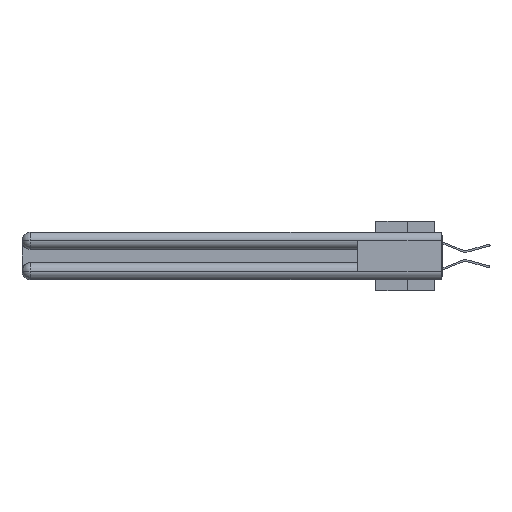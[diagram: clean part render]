
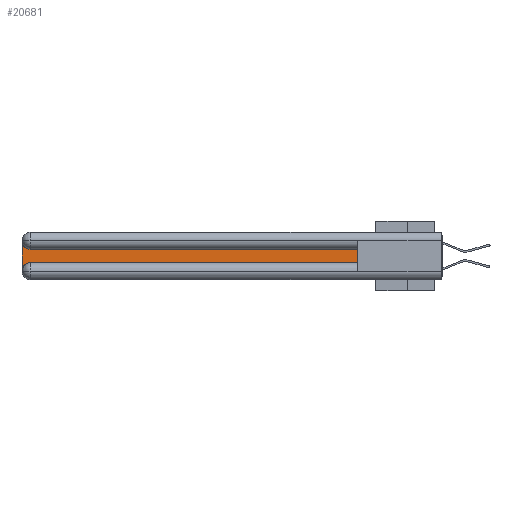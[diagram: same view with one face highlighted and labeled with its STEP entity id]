
A CAD part, left-side view. The second image highlights one B-rep face of the part: STEP entity #20681.
In plain terms, the highlighted planar face has unit normal (-1, 0, 0).
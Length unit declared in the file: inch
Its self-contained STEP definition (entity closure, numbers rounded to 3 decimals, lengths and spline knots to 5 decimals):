
#6 = ORIENTED_EDGE ( 'NONE', *, *, #23174, .T. ) ;
#314 = CIRCLE ( 'NONE', #15308, 0.06 ) ;
#1914 = CARTESIAN_POINT ( 'NONE',  ( 0.075, 2.94, -0.1225 ) ) ;
#2715 = CARTESIAN_POINT ( 'NONE',  ( 0.075, 0.6, -0.2175 ) ) ;
#2827 = DIRECTION ( 'NONE',  ( 1., 0., 0. ) ) ;
#3104 = VERTEX_POINT ( 'NONE', #15729 ) ;
#3452 = CARTESIAN_POINT ( 'NONE',  ( 0.075, 2.94, -0.2775 ) ) ;
#5045 = EDGE_CURVE ( 'NONE', #33990, #6914, #17388, .T. ) ;
#5106 = DIRECTION ( 'NONE',  ( 0., 0., 1. ) ) ;
#5111 = ORIENTED_EDGE ( 'NONE', *, *, #5045, .T. ) ;
#5476 = CARTESIAN_POINT ( 'NONE',  ( 0.075, 0.6, -0.2175 ) ) ;
#5692 = VERTEX_POINT ( 'NONE', #2715 ) ;
#6135 = EDGE_CURVE ( 'NONE', #6914, #3104, #15519, .T. ) ;
#6412 = EDGE_LOOP ( 'NONE', ( #8055, #5111, #7469, #12087, #20218, #6 ) ) ;
#6914 = VERTEX_POINT ( 'NONE', #10956 ) ;
#7347 = DIRECTION ( 'NONE',  ( 0., 1., 0. ) ) ;
#7469 = ORIENTED_EDGE ( 'NONE', *, *, #6135, .T. ) ;
#7632 = EDGE_CURVE ( 'NONE', #3104, #33728, #314, .T. ) ;
#7634 = DIRECTION ( 'NONE',  ( 0., 0., -1. ) ) ;
#8055 = ORIENTED_EDGE ( 'NONE', *, *, #29103, .T. ) ;
#8430 = VERTEX_POINT ( 'NONE', #36486 ) ;
#8545 = VECTOR ( 'NONE', #36013, 39.37008 ) ;
#8676 = FACE_OUTER_BOUND ( 'NONE', #6412, .T. ) ;
#10293 = LINE ( 'NONE', #18914, #13581 ) ;
#10956 = CARTESIAN_POINT ( 'NONE',  ( 0.075, 3., -0.0625 ) ) ;
#11819 = CARTESIAN_POINT ( 'NONE',  ( 0.075, 3., -0.1225 ) ) ;
#12087 = ORIENTED_EDGE ( 'NONE', *, *, #7632, .T. ) ;
#12193 = DIRECTION ( 'NONE',  ( 0., 0., -1. ) ) ;
#13581 = VECTOR ( 'NONE', #7347, 39.37008 ) ;
#15176 = EDGE_CURVE ( 'NONE', #33728, #5692, #24125, .T. ) ;
#15308 = AXIS2_PLACEMENT_3D ( 'NONE', #3452, #24369, #36249 ) ;
#15346 = CARTESIAN_POINT ( 'NONE',  ( 0.075, 0.6, -0.2175 ) ) ;
#15519 = LINE ( 'NONE', #36769, #22599 ) ;
#15729 = CARTESIAN_POINT ( 'NONE',  ( 0.075, 3., -0.2775 ) ) ;
#17388 = CIRCLE ( 'NONE', #31682, 0.06 ) ;
#18914 = CARTESIAN_POINT ( 'NONE',  ( 0.075, 0.6, -0.1225 ) ) ;
#20218 = ORIENTED_EDGE ( 'NONE', *, *, #15176, .T. ) ;
#20681 = ADVANCED_FACE ( 'NONE', ( #8676 ), #21009, .F. ) ;
#21009 = PLANE ( 'NONE',  #36225 ) ;
#22599 = VECTOR ( 'NONE', #12193, 39.37008 ) ;
#23174 = EDGE_CURVE ( 'NONE', #5692, #8430, #23481, .T. ) ;
#23445 = CARTESIAN_POINT ( 'NONE',  ( 0.075, 2.94, -0.2175 ) ) ;
#23481 = LINE ( 'NONE', #5476, #31391 ) ;
#23925 = DIRECTION ( 'NONE',  ( 0., 0., -1. ) ) ;
#24125 = LINE ( 'NONE', #15346, #8545 ) ;
#24369 = DIRECTION ( 'NONE',  ( 1., 0., 0. ) ) ;
#25628 = DIRECTION ( 'NONE',  ( 1., 0., 0. ) ) ;
#28926 = CARTESIAN_POINT ( 'NONE',  ( 0.075, 2.94, -0.0625 ) ) ;
#29103 = EDGE_CURVE ( 'NONE', #8430, #33990, #10293, .T. ) ;
#31391 = VECTOR ( 'NONE', #5106, 39.37008 ) ;
#31682 = AXIS2_PLACEMENT_3D ( 'NONE', #28926, #25628, #7634 ) ;
#33728 = VERTEX_POINT ( 'NONE', #23445 ) ;
#33990 = VERTEX_POINT ( 'NONE', #1914 ) ;
#36013 = DIRECTION ( 'NONE',  ( 0., -1., 0. ) ) ;
#36225 = AXIS2_PLACEMENT_3D ( 'NONE', #11819, #2827, #23925 ) ;
#36249 = DIRECTION ( 'NONE',  ( 0., 0., -1. ) ) ;
#36486 = CARTESIAN_POINT ( 'NONE',  ( 0.075, 0.6, -0.1225 ) ) ;
#36769 = CARTESIAN_POINT ( 'NONE',  ( 0.075, 3., -0.2175 ) ) ;
